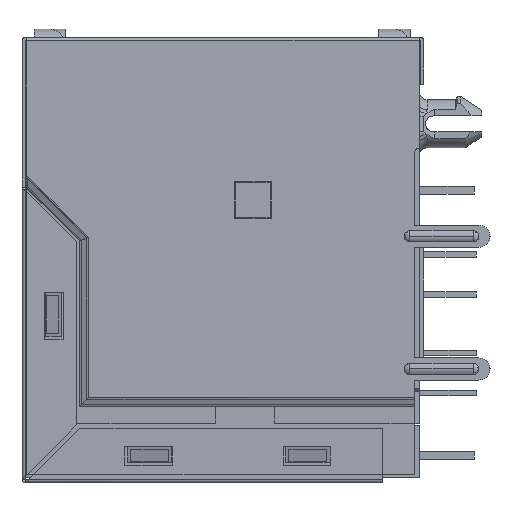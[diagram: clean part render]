
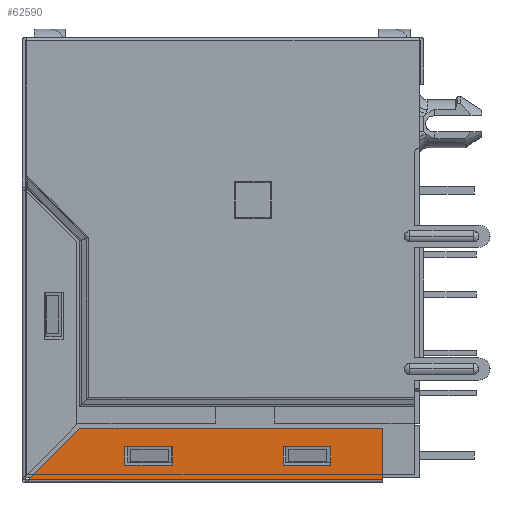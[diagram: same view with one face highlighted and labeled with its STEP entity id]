
A CAD part, left-side view. The second image highlights one B-rep face of the part: STEP entity #62590.
In plain terms, the highlighted planar face has unit normal (-1, 0, 0).
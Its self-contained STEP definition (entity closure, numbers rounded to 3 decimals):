
#4332 = EDGE_CURVE ( 'NONE', #142495, #40222, #67806, .T. ) ;
#6105 = CARTESIAN_POINT ( 'NONE',  ( -31.875, 3.165, -25.58 ) ) ;
#6187 = CARTESIAN_POINT ( 'NONE',  ( -31.875, -6.835, -26.78 ) ) ;
#6684 = CARTESIAN_POINT ( 'NONE',  ( -31.875, 3.165, -26.78 ) ) ;
#6954 = CARTESIAN_POINT ( 'NONE',  ( -31.875, 3.165, -25.58 ) ) ;
#7504 = CARTESIAN_POINT ( 'NONE',  ( -31.875, -10.135, -24.43 ) ) ;
#8053 = ORIENTED_EDGE ( 'NONE', *, *, #21043, .T. ) ;
#11078 = CARTESIAN_POINT ( 'NONE',  ( -31.875, 12.245, -27.67 ) ) ;
#12770 = EDGE_CURVE ( 'NONE', #93878, #104769, #105727, .T. ) ;
#13205 = CARTESIAN_POINT ( 'NONE',  ( -31.875, 9.005, -24.43 ) ) ;
#17146 = CARTESIAN_POINT ( 'NONE',  ( -31.875, 6.165, -25.58 ) ) ;
#17283 = CARTESIAN_POINT ( 'NONE',  ( -31.875, -6.835, -25.58 ) ) ;
#18339 = VERTEX_POINT ( 'NONE', #86434 ) ;
#19457 = EDGE_CURVE ( 'NONE', #23484, #67335, #29640, .T. ) ;
#20819 = VERTEX_POINT ( 'NONE', #56488 ) ;
#21043 = EDGE_CURVE ( 'NONE', #104769, #23484, #70256, .T. ) ;
#21247 = CARTESIAN_POINT ( 'NONE',  ( -31.875, 9.005, -24.43 ) ) ;
#23016 = CARTESIAN_POINT ( 'NONE',  ( -31.875, -3.835, -25.58 ) ) ;
#23484 = VERTEX_POINT ( 'NONE', #60425 ) ;
#27844 = CARTESIAN_POINT ( 'NONE',  ( -31.875, -3.835, -25.58 ) ) ;
#27876 = CARTESIAN_POINT ( 'NONE',  ( -31.875, 6.165, -25.58 ) ) ;
#28289 = CARTESIAN_POINT ( 'NONE',  ( -31.875, -6.835, -26.78 ) ) ;
#29640 = B_SPLINE_CURVE_WITH_KNOTS ( 'NONE', 1,
 ( #28289, #107856 ),
 .UNSPECIFIED., .F., .F.,
 ( 2, 2 ),
 ( 0., 1. ),
 .UNSPECIFIED. ) ;
#34496 = B_SPLINE_CURVE_WITH_KNOTS ( 'NONE', 1,
 ( #120678, #21247 ),
 .UNSPECIFIED., .F., .F.,
 ( 2, 2 ),
 ( 0., 1. ),
 .UNSPECIFIED. ) ;
#40222 = VERTEX_POINT ( 'NONE', #6954 ) ;
#40403 = ORIENTED_EDGE ( 'NONE', *, *, #44010, .F. ) ;
#43916 = CARTESIAN_POINT ( 'NONE',  ( -31.875, -10.135, -24.43 ) ) ;
#44010 = EDGE_CURVE ( 'NONE', #49926, #49597, #72689, .T. ) ;
#47680 = EDGE_CURVE ( 'NONE', #40222, #115790, #84136, .T. ) ;
#47844 = B_SPLINE_CURVE_WITH_KNOTS ( 'NONE', 1,
 ( #104011, #17146 ),
 .UNSPECIFIED., .F., .F.,
 ( 2, 2 ),
 ( 0., 1. ),
 .UNSPECIFIED. ) ;
#49597 = VERTEX_POINT ( 'NONE', #7504 ) ;
#49926 = VERTEX_POINT ( 'NONE', #13205 ) ;
#53696 = ORIENTED_EDGE ( 'NONE', *, *, #12770, .T. ) ;
#54866 = EDGE_LOOP ( 'NONE', ( #89032, #64312, #108171, #95467 ) ) ;
#56488 = CARTESIAN_POINT ( 'NONE',  ( -31.875, 6.165, -26.78 ) ) ;
#56495 = ORIENTED_EDGE ( 'NONE', *, *, #101926, .T. ) ;
#60425 = CARTESIAN_POINT ( 'NONE',  ( -31.875, -6.835, -26.78 ) ) ;
#61088 = B_SPLINE_CURVE_WITH_KNOTS ( 'NONE', 1,
 ( #99009, #76316 ),
 .UNSPECIFIED., .F., .F.,
 ( 2, 2 ),
 ( 0., 1. ),
 .UNSPECIFIED. ) ;
#62590 = ADVANCED_FACE ( 'NONE', ( #127702, #94857, #120780 ), #116081, .T. ) ;
#64312 = ORIENTED_EDGE ( 'NONE', *, *, #4332, .T. ) ;
#64687 = CARTESIAN_POINT ( 'NONE',  ( -31.875, -10.135, -27.67 ) ) ;
#65654 = ORIENTED_EDGE ( 'NONE', *, *, #67138, .T. ) ;
#67138 = EDGE_CURVE ( 'NONE', #67335, #93878, #102743, .T. ) ;
#67335 = VERTEX_POINT ( 'NONE', #108387 ) ;
#67806 = B_SPLINE_CURVE_WITH_KNOTS ( 'NONE', 1,
 ( #27876, #6105 ),
 .UNSPECIFIED., .F., .F.,
 ( 2, 2 ),
 ( 0., 1. ),
 .UNSPECIFIED. ) ;
#70256 = B_SPLINE_CURVE_WITH_KNOTS ( 'NONE', 1,
 ( #17283, #6187 ),
 .UNSPECIFIED., .F., .F.,
 ( 2, 2 ),
 ( 0., 1. ),
 .UNSPECIFIED. ) ;
#71521 = B_SPLINE_CURVE_WITH_KNOTS ( 'NONE', 1,
 ( #131246, #64687 ),
 .UNSPECIFIED., .F., .F.,
 ( 2, 2 ),
 ( 0., 1. ),
 .UNSPECIFIED. ) ;
#71634 = CARTESIAN_POINT ( 'NONE',  ( -31.875, 12.693, -27.766 ) ) ;
#72689 = B_SPLINE_CURVE_WITH_KNOTS ( 'NONE', 1,
 ( #100306, #43916 ),
 .UNSPECIFIED., .F., .F.,
 ( 2, 2 ),
 ( 0., 1. ),
 .UNSPECIFIED. ) ;
#74390 = EDGE_CURVE ( 'NONE', #49597, #18339, #61088, .T. ) ;
#74805 = B_SPLINE_CURVE_WITH_KNOTS ( 'NONE', 1,
 ( #6684, #83915 ),
 .UNSPECIFIED., .F., .F.,
 ( 2, 2 ),
 ( 0., 1. ),
 .UNSPECIFIED. ) ;
#76316 = CARTESIAN_POINT ( 'NONE',  ( -31.875, -10.135, -27.67 ) ) ;
#76897 = EDGE_LOOP ( 'NONE', ( #122033, #56495, #89445, #40403 ) ) ;
#77061 = EDGE_LOOP ( 'NONE', ( #65654, #53696, #8053, #77923 ) ) ;
#77923 = ORIENTED_EDGE ( 'NONE', *, *, #19457, .T. ) ;
#78528 = EDGE_CURVE ( 'NONE', #20819, #142495, #47844, .T. ) ;
#83871 = CARTESIAN_POINT ( 'NONE',  ( -31.875, -3.835, -26.78 ) ) ;
#83915 = CARTESIAN_POINT ( 'NONE',  ( -31.875, 6.165, -26.78 ) ) ;
#84136 = B_SPLINE_CURVE_WITH_KNOTS ( 'NONE', 1,
 ( #87943, #110670 ),
 .UNSPECIFIED., .F., .F.,
 ( 2, 2 ),
 ( 0., 1. ),
 .UNSPECIFIED. ) ;
#84497 = CARTESIAN_POINT ( 'NONE',  ( -31.875, 6.165, -25.58 ) ) ;
#86434 = CARTESIAN_POINT ( 'NONE',  ( -31.875, -10.135, -27.67 ) ) ;
#87340 = AXIS2_PLACEMENT_3D ( 'NONE', #71634, #93341, #117515 ) ;
#87943 = CARTESIAN_POINT ( 'NONE',  ( -31.875, 3.165, -25.58 ) ) ;
#89032 = ORIENTED_EDGE ( 'NONE', *, *, #78528, .T. ) ;
#89445 = ORIENTED_EDGE ( 'NONE', *, *, #74390, .F. ) ;
#92897 = EDGE_CURVE ( 'NONE', #108262, #49926, #34496, .T. ) ;
#93341 = DIRECTION ( 'NONE',  ( -1., 0., 0. ) ) ;
#93878 = VERTEX_POINT ( 'NONE', #27844 ) ;
#94857 = FACE_BOUND ( 'NONE', #54866, .T. ) ;
#95467 = ORIENTED_EDGE ( 'NONE', *, *, #130133, .T. ) ;
#99009 = CARTESIAN_POINT ( 'NONE',  ( -31.875, -10.135, -24.43 ) ) ;
#100306 = CARTESIAN_POINT ( 'NONE',  ( -31.875, 9.005, -24.43 ) ) ;
#100757 = CARTESIAN_POINT ( 'NONE',  ( -31.875, -3.835, -25.58 ) ) ;
#101926 = EDGE_CURVE ( 'NONE', #108262, #18339, #71521, .T. ) ;
#102743 = B_SPLINE_CURVE_WITH_KNOTS ( 'NONE', 1,
 ( #83871, #23016 ),
 .UNSPECIFIED., .F., .F.,
 ( 2, 2 ),
 ( 0., 1. ),
 .UNSPECIFIED. ) ;
#104011 = CARTESIAN_POINT ( 'NONE',  ( -31.875, 6.165, -26.78 ) ) ;
#104769 = VERTEX_POINT ( 'NONE', #110084 ) ;
#105727 = B_SPLINE_CURVE_WITH_KNOTS ( 'NONE', 1,
 ( #100757, #112835 ),
 .UNSPECIFIED., .F., .F.,
 ( 2, 2 ),
 ( 0., 1. ),
 .UNSPECIFIED. ) ;
#107856 = CARTESIAN_POINT ( 'NONE',  ( -31.875, -3.835, -26.78 ) ) ;
#108171 = ORIENTED_EDGE ( 'NONE', *, *, #47680, .T. ) ;
#108262 = VERTEX_POINT ( 'NONE', #11078 ) ;
#108387 = CARTESIAN_POINT ( 'NONE',  ( -31.875, -3.835, -26.78 ) ) ;
#110084 = CARTESIAN_POINT ( 'NONE',  ( -31.875, -6.835, -25.58 ) ) ;
#110670 = CARTESIAN_POINT ( 'NONE',  ( -31.875, 3.165, -26.78 ) ) ;
#111631 = CARTESIAN_POINT ( 'NONE',  ( -31.875, 3.165, -26.78 ) ) ;
#112835 = CARTESIAN_POINT ( 'NONE',  ( -31.875, -6.835, -25.58 ) ) ;
#115790 = VERTEX_POINT ( 'NONE', #111631 ) ;
#116081 = PLANE ( 'NONE',  #87340 ) ;
#117515 = DIRECTION ( 'NONE',  ( 0., -1., 0. ) ) ;
#120678 = CARTESIAN_POINT ( 'NONE',  ( -31.875, 12.245, -27.67 ) ) ;
#120780 = FACE_BOUND ( 'NONE', #77061, .T. ) ;
#122033 = ORIENTED_EDGE ( 'NONE', *, *, #92897, .F. ) ;
#127702 = FACE_OUTER_BOUND ( 'NONE', #76897, .T. ) ;
#130133 = EDGE_CURVE ( 'NONE', #115790, #20819, #74805, .T. ) ;
#131246 = CARTESIAN_POINT ( 'NONE',  ( -31.875, 12.245, -27.67 ) ) ;
#142495 = VERTEX_POINT ( 'NONE', #84497 ) ;
